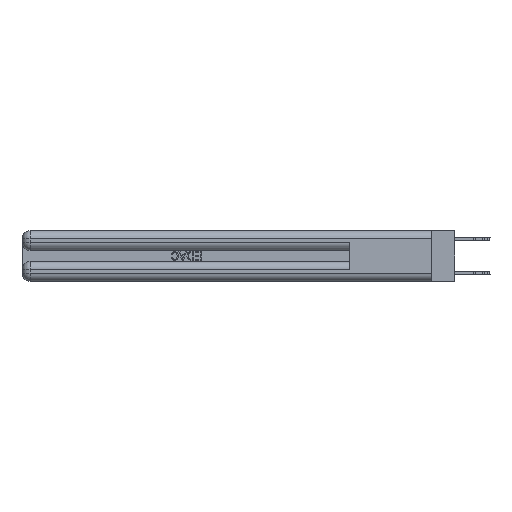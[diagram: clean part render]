
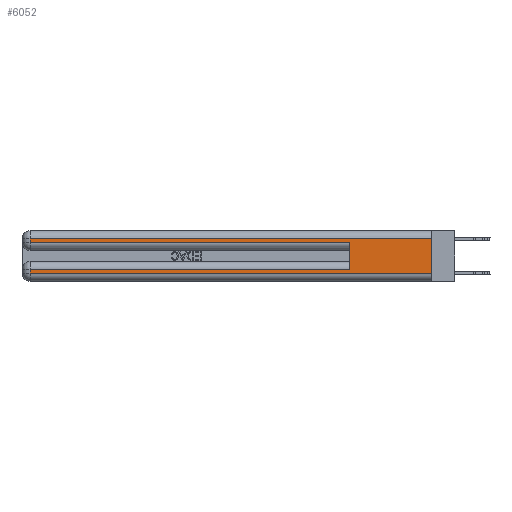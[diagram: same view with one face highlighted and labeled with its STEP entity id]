
A CAD part, left-side view. The second image highlights one B-rep face of the part: STEP entity #6052.
In plain terms, the highlighted planar face has unit normal (-1, 0, 0).
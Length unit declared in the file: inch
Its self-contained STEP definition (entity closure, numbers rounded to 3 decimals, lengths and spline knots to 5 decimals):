
#1005 = CARTESIAN_POINT ( 'NONE',  ( 0., 2.94, 0.06 ) ) ;
#2435 = LINE ( 'NONE', #24359, #16433 ) ;
#3281 = LINE ( 'NONE', #13794, #6004 ) ;
#3932 = CARTESIAN_POINT ( 'NONE',  ( 0., 2.94, 0.085 ) ) ;
#4563 = LINE ( 'NONE', #12623, #15278 ) ;
#5043 = LINE ( 'NONE', #26260, #29310 ) ;
#5103 = CARTESIAN_POINT ( 'NONE',  ( 0., 0.6, 0.085 ) ) ;
#5257 = VERTEX_POINT ( 'NONE', #27378 ) ;
#5377 = VERTEX_POINT ( 'NONE', #34211 ) ;
#5533 = EDGE_CURVE ( 'NONE', #26187, #26868, #2435, .T. ) ;
#5580 = ORIENTED_EDGE ( 'NONE', *, *, #5533, .T. ) ;
#6004 = VECTOR ( 'NONE', #16785, 39.37008 ) ;
#6052 = ADVANCED_FACE ( 'NONE', ( #12538 ), #9748, .F. ) ;
#6469 = EDGE_CURVE ( 'NONE', #26187, #11976, #4563, .T. ) ;
#6930 = AXIS2_PLACEMENT_3D ( 'NONE', #23234, #20411, #31144 ) ;
#8230 = EDGE_CURVE ( 'NONE', #5377, #11976, #15523, .T. ) ;
#8677 = LINE ( 'NONE', #13918, #20890 ) ;
#9748 = PLANE ( 'NONE',  #6930 ) ;
#10237 = EDGE_CURVE ( 'NONE', #32964, #5257, #10928, .T. ) ;
#10266 = VERTEX_POINT ( 'NONE', #33708 ) ;
#10869 = CARTESIAN_POINT ( 'NONE',  ( 0., 2.94, 0.31 ) ) ;
#10928 = LINE ( 'NONE', #19315, #26095 ) ;
#11976 = VERTEX_POINT ( 'NONE', #21744 ) ;
#11977 = VECTOR ( 'NONE', #26223, 39.37008 ) ;
#12538 = FACE_OUTER_BOUND ( 'NONE', #25581, .T. ) ;
#12623 = CARTESIAN_POINT ( 'NONE',  ( 0., 0.6, 0.145 ) ) ;
#13156 = DIRECTION ( 'NONE',  ( 0., 0., -1. ) ) ;
#13794 = CARTESIAN_POINT ( 'NONE',  ( 0., 2.94, 0.37 ) ) ;
#13918 = CARTESIAN_POINT ( 'NONE',  ( 0., 0., 0.31 ) ) ;
#15278 = VECTOR ( 'NONE', #20508, 39.37008 ) ;
#15523 = LINE ( 'NONE', #20948, #11977 ) ;
#15765 = ORIENTED_EDGE ( 'NONE', *, *, #25009, .T. ) ;
#16433 = VECTOR ( 'NONE', #31927, 39.37008 ) ;
#16785 = DIRECTION ( 'NONE',  ( 0., 0., -1. ) ) ;
#17138 = ORIENTED_EDGE ( 'NONE', *, *, #26145, .F. ) ;
#18971 = ORIENTED_EDGE ( 'NONE', *, *, #6469, .F. ) ;
#19035 = VERTEX_POINT ( 'NONE', #10869 ) ;
#19315 = CARTESIAN_POINT ( 'NONE',  ( 0., 0., 0.06 ) ) ;
#20411 = DIRECTION ( 'NONE',  ( 1., 0., 0. ) ) ;
#20508 = DIRECTION ( 'NONE',  ( 0., 0., 1. ) ) ;
#20890 = VECTOR ( 'NONE', #31243, 39.37008 ) ;
#20948 = CARTESIAN_POINT ( 'NONE',  ( 0., 0., 0.285 ) ) ;
#21744 = CARTESIAN_POINT ( 'NONE',  ( 0., 0.6, 0.285 ) ) ;
#23234 = CARTESIAN_POINT ( 'NONE',  ( 0., 0., 0.37 ) ) ;
#23343 = LINE ( 'NONE', #23690, #23426 ) ;
#23426 = VECTOR ( 'NONE', #13156, 39.37008 ) ;
#23690 = CARTESIAN_POINT ( 'NONE',  ( 0., 0., 0.37 ) ) ;
#24359 = CARTESIAN_POINT ( 'NONE',  ( 0., 0., 0.085 ) ) ;
#25009 = EDGE_CURVE ( 'NONE', #26868, #32964, #3281, .T. ) ;
#25581 = EDGE_LOOP ( 'NONE', ( #17138, #27422, #27346, #33661, #18971, #5580, #15765, #28109 ) ) ;
#25914 = DIRECTION ( 'NONE',  ( 0., 0., -1. ) ) ;
#26095 = VECTOR ( 'NONE', #27403, 39.37008 ) ;
#26145 = EDGE_CURVE ( 'NONE', #10266, #5257, #23343, .T. ) ;
#26187 = VERTEX_POINT ( 'NONE', #5103 ) ;
#26223 = DIRECTION ( 'NONE',  ( 0., -1., 0. ) ) ;
#26260 = CARTESIAN_POINT ( 'NONE',  ( 0., 2.94, 0.37 ) ) ;
#26868 = VERTEX_POINT ( 'NONE', #3932 ) ;
#27346 = ORIENTED_EDGE ( 'NONE', *, *, #31837, .T. ) ;
#27378 = CARTESIAN_POINT ( 'NONE',  ( 0., 0., 0.06 ) ) ;
#27403 = DIRECTION ( 'NONE',  ( 0., -1., 0. ) ) ;
#27422 = ORIENTED_EDGE ( 'NONE', *, *, #31248, .T. ) ;
#28109 = ORIENTED_EDGE ( 'NONE', *, *, #10237, .T. ) ;
#29310 = VECTOR ( 'NONE', #25914, 39.37008 ) ;
#31144 = DIRECTION ( 'NONE',  ( 0., 0., -1. ) ) ;
#31243 = DIRECTION ( 'NONE',  ( 0., 1., 0. ) ) ;
#31248 = EDGE_CURVE ( 'NONE', #10266, #19035, #8677, .T. ) ;
#31837 = EDGE_CURVE ( 'NONE', #19035, #5377, #5043, .T. ) ;
#31927 = DIRECTION ( 'NONE',  ( 0., 1., 0. ) ) ;
#32964 = VERTEX_POINT ( 'NONE', #1005 ) ;
#33661 = ORIENTED_EDGE ( 'NONE', *, *, #8230, .T. ) ;
#33708 = CARTESIAN_POINT ( 'NONE',  ( 0., 0., 0.31 ) ) ;
#34211 = CARTESIAN_POINT ( 'NONE',  ( 0., 2.94, 0.285 ) ) ;
